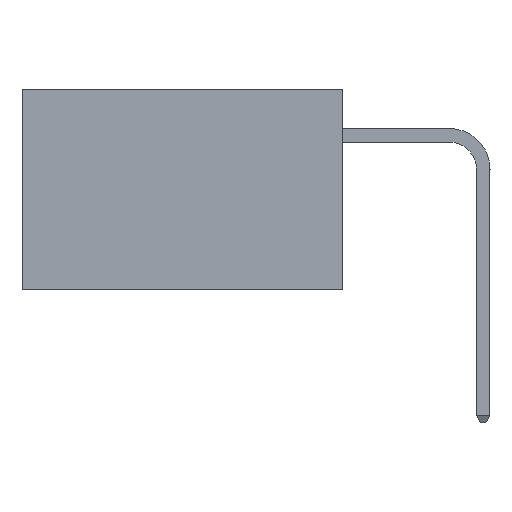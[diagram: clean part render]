
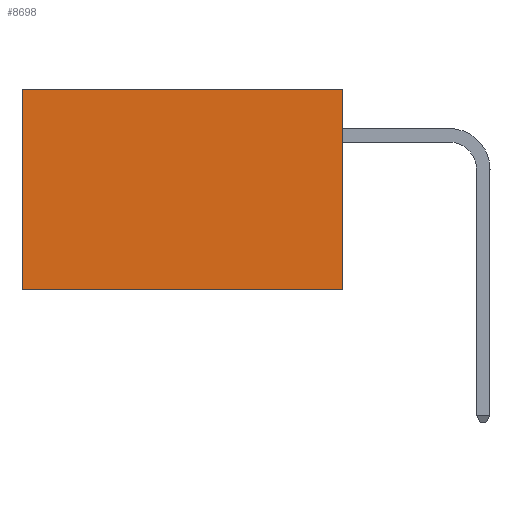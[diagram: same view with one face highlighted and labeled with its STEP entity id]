
A CAD part, left-side view. The second image highlights one B-rep face of the part: STEP entity #8698.
In plain terms, the highlighted planar face has unit normal (-1, 0, 0).
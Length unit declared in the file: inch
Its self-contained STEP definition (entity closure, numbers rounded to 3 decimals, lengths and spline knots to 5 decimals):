
#217 = CARTESIAN_POINT ( 'NONE',  ( 0.277, 0., 0. ) ) ;
#2044 = CARTESIAN_POINT ( 'NONE',  ( 0.277, 0., -0.37 ) ) ;
#2704 = EDGE_CURVE ( 'NONE', #14538, #27648, #22774, .T. ) ;
#3611 = CARTESIAN_POINT ( 'NONE',  ( 0.277, 0., -0.37 ) ) ;
#3935 = DIRECTION ( 'NONE',  ( 0., 1., 0. ) ) ;
#4277 = EDGE_LOOP ( 'NONE', ( #5352, #10186, #20187, #16079 ) ) ;
#4390 = VECTOR ( 'NONE', #5445, 39.37008 ) ;
#5352 = ORIENTED_EDGE ( 'NONE', *, *, #27054, .T. ) ;
#5445 = DIRECTION ( 'NONE',  ( 0., 0., -1. ) ) ;
#6845 = EDGE_CURVE ( 'NONE', #25738, #14538, #11044, .T. ) ;
#7660 = CARTESIAN_POINT ( 'NONE',  ( 0.277, 0.59, -0.37 ) ) ;
#8212 = CARTESIAN_POINT ( 'NONE',  ( 0.277, 0., 0. ) ) ;
#8698 = ADVANCED_FACE ( 'NONE', ( #15214 ), #11613, .F. ) ;
#9558 = CARTESIAN_POINT ( 'NONE',  ( 0.277, 0.59, 0. ) ) ;
#9798 = CARTESIAN_POINT ( 'NONE',  ( 0.277, 0.59, -0.37 ) ) ;
#10186 = ORIENTED_EDGE ( 'NONE', *, *, #2704, .F. ) ;
#10875 = LINE ( 'NONE', #7660, #24058 ) ;
#11044 = LINE ( 'NONE', #17908, #4390 ) ;
#11613 = PLANE ( 'NONE',  #24247 ) ;
#13160 = VERTEX_POINT ( 'NONE', #9558 ) ;
#14538 = VERTEX_POINT ( 'NONE', #2044 ) ;
#15214 = FACE_OUTER_BOUND ( 'NONE', #4277, .T. ) ;
#16079 = ORIENTED_EDGE ( 'NONE', *, *, #31032, .T. ) ;
#16216 = VECTOR ( 'NONE', #3935, 39.37008 ) ;
#16616 = DIRECTION ( 'NONE',  ( 0., 0., -1. ) ) ;
#16842 = LINE ( 'NONE', #8212, #22602 ) ;
#17908 = CARTESIAN_POINT ( 'NONE',  ( 0.277, 0., -0.37 ) ) ;
#20187 = ORIENTED_EDGE ( 'NONE', *, *, #6845, .F. ) ;
#22602 = VECTOR ( 'NONE', #27972, 39.37008 ) ;
#22774 = LINE ( 'NONE', #3611, #16216 ) ;
#24058 = VECTOR ( 'NONE', #24982, 39.37008 ) ;
#24247 = AXIS2_PLACEMENT_3D ( 'NONE', #28859, #31292, #16616 ) ;
#24982 = DIRECTION ( 'NONE',  ( 0., 0., -1. ) ) ;
#25738 = VERTEX_POINT ( 'NONE', #217 ) ;
#27054 = EDGE_CURVE ( 'NONE', #13160, #27648, #10875, .T. ) ;
#27648 = VERTEX_POINT ( 'NONE', #9798 ) ;
#27972 = DIRECTION ( 'NONE',  ( 0., 1., 0. ) ) ;
#28859 = CARTESIAN_POINT ( 'NONE',  ( 0.277, 0., -0.37 ) ) ;
#31032 = EDGE_CURVE ( 'NONE', #25738, #13160, #16842, .T. ) ;
#31292 = DIRECTION ( 'NONE',  ( 1., 0., 0. ) ) ;
